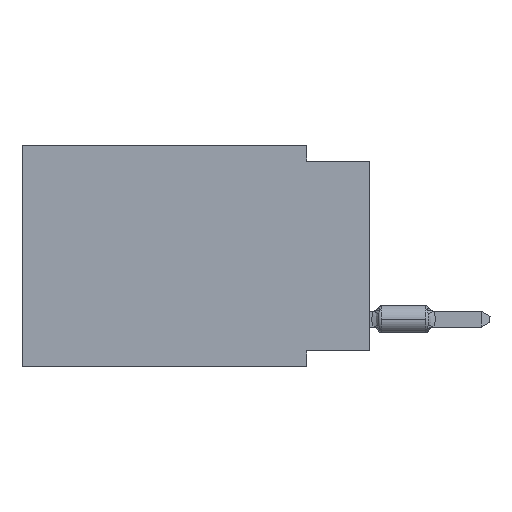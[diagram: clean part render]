
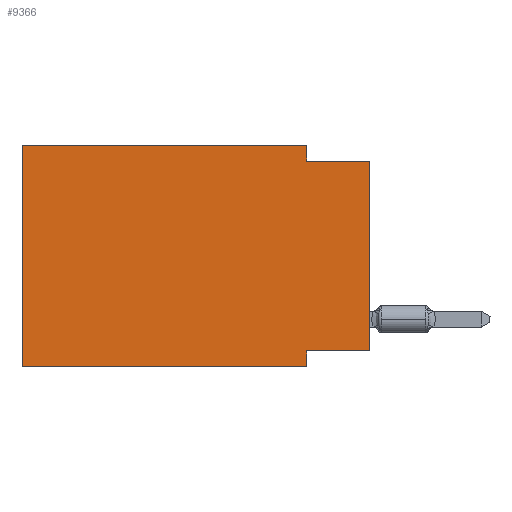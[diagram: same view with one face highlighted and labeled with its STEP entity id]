
A CAD part, left-side view. The second image highlights one B-rep face of the part: STEP entity #9366.
In plain terms, the highlighted planar face has unit normal (-1, 0, 0).
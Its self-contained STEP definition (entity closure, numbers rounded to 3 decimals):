
#576 = EDGE_CURVE ( 'NONE', #84521, #61870, #91247, .T. ) ;
#3121 = DIRECTION ( 'NONE',  ( 1., 0., 0. ) ) ;
#6441 = EDGE_CURVE ( 'NONE', #39639, #69648, #15567, .T. ) ;
#9366 = ADVANCED_FACE ( 'NONE', ( #84700 ), #92992, .F. ) ;
#11167 = ORIENTED_EDGE ( 'NONE', *, *, #28687, .F. ) ;
#15567 = LINE ( 'NONE', #60003, #76230 ) ;
#15782 = LINE ( 'NONE', #24058, #35832 ) ;
#16268 = VERTEX_POINT ( 'NONE', #18016 ) ;
#17807 = CARTESIAN_POINT ( 'NONE',  ( 0., 13.97, 0. ) ) ;
#18016 = CARTESIAN_POINT ( 'NONE',  ( 0., 2.54, -8.255 ) ) ;
#18298 = CARTESIAN_POINT ( 'NONE',  ( 0., 2.54, -0.635 ) ) ;
#18881 = CARTESIAN_POINT ( 'NONE',  ( 0., 13.97, 0. ) ) ;
#21314 = VECTOR ( 'NONE', #30904, 1000. ) ;
#22855 = EDGE_CURVE ( 'NONE', #16268, #74394, #84122, .T. ) ;
#24058 = CARTESIAN_POINT ( 'NONE',  ( 0., 13.97, -8.89 ) ) ;
#26003 = ORIENTED_EDGE ( 'NONE', *, *, #22855, .F. ) ;
#28687 = EDGE_CURVE ( 'NONE', #34141, #84521, #78921, .T. ) ;
#28736 = VECTOR ( 'NONE', #76604, 1000. ) ;
#30904 = DIRECTION ( 'NONE',  ( 0., 0., -1. ) ) ;
#34141 = VERTEX_POINT ( 'NONE', #37923 ) ;
#34475 = DIRECTION ( 'NONE',  ( 0., 0., 1. ) ) ;
#35832 = VECTOR ( 'NONE', #45574, 1000. ) ;
#37923 = CARTESIAN_POINT ( 'NONE',  ( 0., 13.97, -8.89 ) ) ;
#38061 = CARTESIAN_POINT ( 'NONE',  ( 0., 0., -0.635 ) ) ;
#39639 = VERTEX_POINT ( 'NONE', #74789 ) ;
#39826 = ORIENTED_EDGE ( 'NONE', *, *, #71511, .F. ) ;
#40016 = ORIENTED_EDGE ( 'NONE', *, *, #576, .F. ) ;
#40226 = ORIENTED_EDGE ( 'NONE', *, *, #76365, .F. ) ;
#43011 = DIRECTION ( 'NONE',  ( 0., -1., 0. ) ) ;
#44592 = CARTESIAN_POINT ( 'NONE',  ( 0., 13.97, 0. ) ) ;
#45574 = DIRECTION ( 'NONE',  ( 0., -1., 0. ) ) ;
#45855 = CARTESIAN_POINT ( 'NONE',  ( 0., 13.97, 0. ) ) ;
#48940 = LINE ( 'NONE', #64051, #54834 ) ;
#50081 = CARTESIAN_POINT ( 'NONE',  ( 0., 2.54, -8.89 ) ) ;
#52087 = VERTEX_POINT ( 'NONE', #18298 ) ;
#52119 = LINE ( 'NONE', #96534, #91593 ) ;
#53317 = EDGE_LOOP ( 'NONE', ( #70391, #94785, #39826, #40016, #11167, #79457, #26003, #40226 ) ) ;
#54834 = VECTOR ( 'NONE', #43011, 1000. ) ;
#56220 = AXIS2_PLACEMENT_3D ( 'NONE', #17807, #3121, #62740 ) ;
#60003 = CARTESIAN_POINT ( 'NONE',  ( 0., 0., 0. ) ) ;
#61870 = VERTEX_POINT ( 'NONE', #87497 ) ;
#62740 = DIRECTION ( 'NONE',  ( 0., 0., -1. ) ) ;
#64051 = CARTESIAN_POINT ( 'NONE',  ( 0., 0., -0.635 ) ) ;
#64136 = EDGE_CURVE ( 'NONE', #34141, #74394, #15782, .T. ) ;
#68292 = DIRECTION ( 'NONE',  ( 0., 0., 1. ) ) ;
#69180 = DIRECTION ( 'NONE',  ( 0., 0., -1. ) ) ;
#69648 = VERTEX_POINT ( 'NONE', #38061 ) ;
#70391 = ORIENTED_EDGE ( 'NONE', *, *, #6441, .T. ) ;
#71511 = EDGE_CURVE ( 'NONE', #61870, #52087, #82364, .T. ) ;
#74394 = VERTEX_POINT ( 'NONE', #50081 ) ;
#74789 = CARTESIAN_POINT ( 'NONE',  ( 0., 0., -8.255 ) ) ;
#76230 = VECTOR ( 'NONE', #68292, 1000. ) ;
#76365 = EDGE_CURVE ( 'NONE', #39639, #16268, #52119, .T. ) ;
#76604 = DIRECTION ( 'NONE',  ( 0., -1., 0. ) ) ;
#78921 = LINE ( 'NONE', #18881, #95436 ) ;
#79457 = ORIENTED_EDGE ( 'NONE', *, *, #64136, .T. ) ;
#80836 = EDGE_CURVE ( 'NONE', #52087, #69648, #48940, .T. ) ;
#80841 = VECTOR ( 'NONE', #69180, 1000. ) ;
#82364 = LINE ( 'NONE', #91148, #80841 ) ;
#83149 = CARTESIAN_POINT ( 'NONE',  ( 0., 2.54, -8.89 ) ) ;
#84122 = LINE ( 'NONE', #83149, #21314 ) ;
#84521 = VERTEX_POINT ( 'NONE', #44592 ) ;
#84700 = FACE_OUTER_BOUND ( 'NONE', #53317, .T. ) ;
#87497 = CARTESIAN_POINT ( 'NONE',  ( 0., 2.54, 0. ) ) ;
#90159 = DIRECTION ( 'NONE',  ( 0., 1., 0. ) ) ;
#91148 = CARTESIAN_POINT ( 'NONE',  ( 0., 2.54, 0. ) ) ;
#91247 = LINE ( 'NONE', #45855, #28736 ) ;
#91593 = VECTOR ( 'NONE', #90159, 1000. ) ;
#92992 = PLANE ( 'NONE',  #56220 ) ;
#94785 = ORIENTED_EDGE ( 'NONE', *, *, #80836, .F. ) ;
#95436 = VECTOR ( 'NONE', #34475, 1000. ) ;
#96534 = CARTESIAN_POINT ( 'NONE',  ( 0., 0., -8.255 ) ) ;
